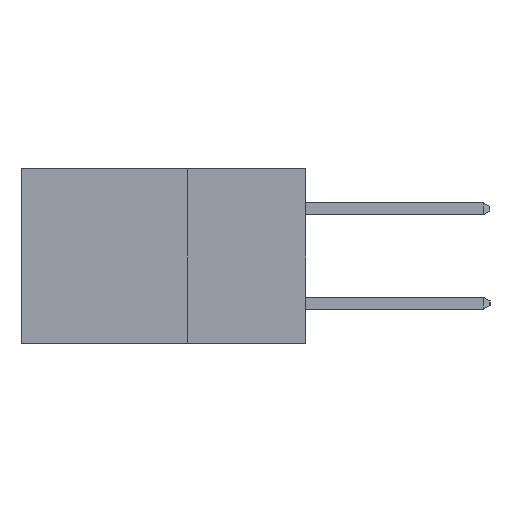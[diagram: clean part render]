
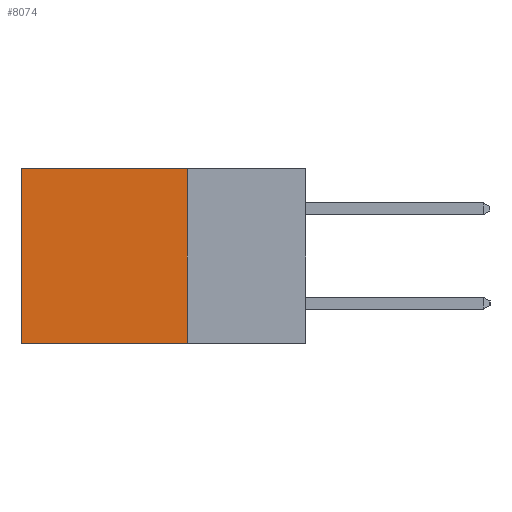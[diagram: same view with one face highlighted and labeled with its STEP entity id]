
A CAD part, left-side view. The second image highlights one B-rep face of the part: STEP entity #8074.
In plain terms, the highlighted planar face has unit normal (-1, 0, 0).
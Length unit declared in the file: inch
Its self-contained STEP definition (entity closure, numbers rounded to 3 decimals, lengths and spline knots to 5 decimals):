
#328 = DIRECTION ( 'NONE',  ( 0., 0., -1. ) ) ;
#815 = FACE_OUTER_BOUND ( 'NONE', #9727, .T. ) ;
#1104 = DIRECTION ( 'NONE',  ( 0., 0., -1. ) ) ;
#1246 = VERTEX_POINT ( 'NONE', #6669 ) ;
#1481 = EDGE_CURVE ( 'NONE', #7452, #5221, #11087, .T. ) ;
#1932 = CARTESIAN_POINT ( 'NONE',  ( 0.2615, 0.25, -0.37 ) ) ;
#2117 = LINE ( 'NONE', #1932, #10944 ) ;
#2877 = ORIENTED_EDGE ( 'NONE', *, *, #6167, .F. ) ;
#3434 = DIRECTION ( 'NONE',  ( 0., 1., 0. ) ) ;
#3560 = EDGE_CURVE ( 'NONE', #1246, #8993, #7012, .T. ) ;
#3879 = CARTESIAN_POINT ( 'NONE',  ( 0.2615, 0.25, -0.37 ) ) ;
#4380 = CARTESIAN_POINT ( 'NONE',  ( 0.2615, 0.25, 0. ) ) ;
#4641 = VECTOR ( 'NONE', #6673, 39.37008 ) ;
#5192 = ORIENTED_EDGE ( 'NONE', *, *, #1481, .T. ) ;
#5221 = VERTEX_POINT ( 'NONE', #10165 ) ;
#5597 = DIRECTION ( 'NONE',  ( 1., 0., 0. ) ) ;
#6167 = EDGE_CURVE ( 'NONE', #7452, #1246, #2117, .T. ) ;
#6544 = CARTESIAN_POINT ( 'NONE',  ( 0.2615, 0.25, 0. ) ) ;
#6669 = CARTESIAN_POINT ( 'NONE',  ( 0.2615, 0.25, -0.37 ) ) ;
#6673 = DIRECTION ( 'NONE',  ( 0., 1., 0. ) ) ;
#6791 = AXIS2_PLACEMENT_3D ( 'NONE', #8954, #5597, #328 ) ;
#7012 = LINE ( 'NONE', #3879, #8716 ) ;
#7111 = CARTESIAN_POINT ( 'NONE',  ( 0.2615, 0.6, -0.37 ) ) ;
#7201 = ORIENTED_EDGE ( 'NONE', *, *, #8507, .T. ) ;
#7252 = VECTOR ( 'NONE', #8770, 39.37008 ) ;
#7452 = VERTEX_POINT ( 'NONE', #6544 ) ;
#7530 = LINE ( 'NONE', #7111, #7252 ) ;
#8074 = ADVANCED_FACE ( 'NONE', ( #815 ), #10674, .F. ) ;
#8507 = EDGE_CURVE ( 'NONE', #5221, #8993, #7530, .T. ) ;
#8716 = VECTOR ( 'NONE', #3434, 39.37008 ) ;
#8770 = DIRECTION ( 'NONE',  ( 0., 0., -1. ) ) ;
#8954 = CARTESIAN_POINT ( 'NONE',  ( 0.2615, 0.25, -0.37 ) ) ;
#8993 = VERTEX_POINT ( 'NONE', #10722 ) ;
#9398 = ORIENTED_EDGE ( 'NONE', *, *, #3560, .F. ) ;
#9727 = EDGE_LOOP ( 'NONE', ( #7201, #9398, #2877, #5192 ) ) ;
#10165 = CARTESIAN_POINT ( 'NONE',  ( 0.2615, 0.6, 0. ) ) ;
#10674 = PLANE ( 'NONE',  #6791 ) ;
#10722 = CARTESIAN_POINT ( 'NONE',  ( 0.2615, 0.6, -0.37 ) ) ;
#10944 = VECTOR ( 'NONE', #1104, 39.37008 ) ;
#11087 = LINE ( 'NONE', #4380, #4641 ) ;
